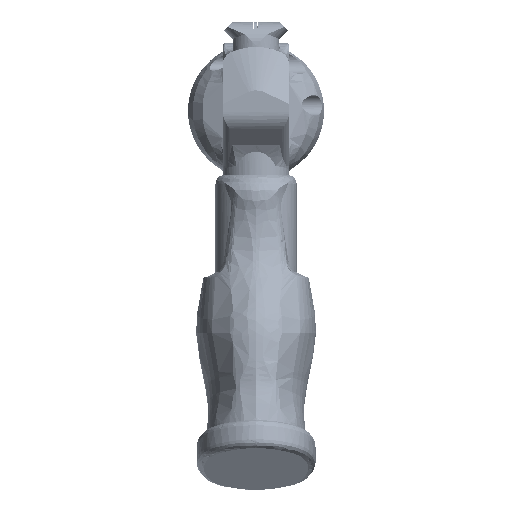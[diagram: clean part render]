
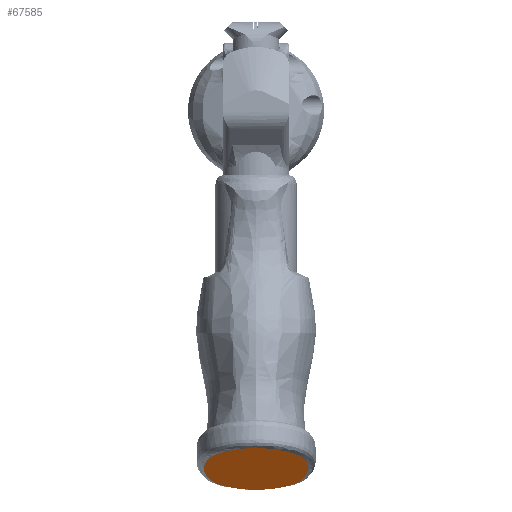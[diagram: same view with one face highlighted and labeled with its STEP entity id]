
A CAD part, left-side view. The second image highlights one B-rep face of the part: STEP entity #67585.
In plain terms, the highlighted planar face has unit normal (-0.259, 0, -0.966).
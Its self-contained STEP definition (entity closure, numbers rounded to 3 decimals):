
#2173=B_SPLINE_CURVE_WITH_KNOTS('',3,(#161349,#161350,#161351,#161352,#161353,
#161354,#161355,#161356,#161357,#161358,#161359,#161360,#161361,#161362,
#161363,#161364,#161365,#161366,#161367,#161368,#161369,#161370,#161371,
#161372,#161373,#161374,#161375,#161376,#161377,#161378,#161379,#161380,
#161381,#161382,#161383,#161384,#161385,#161386,#161387,#161388,#161389,
#161390,#161391),.UNSPECIFIED.,.F.,.F.,(4,2,2,1,1,2,2,2,2,2,1,2,2,2,2,2,
1,2,2,2,1,2,2,4),(0.006,0.019,0.572,
0.597,0.912,1.167,1.831,2.109,
2.578,3.454,3.481,3.884,4.134,
4.709,4.967,5.471,5.557,6.204,
6.731,6.892,6.95,7.028,7.341,
7.351),.UNSPECIFIED.);
#2178=B_SPLINE_CURVE_WITH_KNOTS('',3,(#162170,#162171,#162172,#162173,#162174,
#162175,#162176,#162177,#162178,#162179,#162180,#162181,#162182,#162183,
#162184,#162185,#162186,#162187,#162188,#162189,#162190,#162191,#162192,
#162193,#162194,#162195,#162196,#162197,#162198,#162199,#162200,#162201,
#162202,#162203,#162204,#162205,#162206,#162207,#162208,#162209),
 .UNSPECIFIED.,.F.,.F.,(4,2,2,2,1,2,2,1,2,2,2,1,2,2,2,1,1,2,1,2,2,2,4),
(0.005,0.015,0.356,0.55,
1.005,1.346,1.422,1.811,2.103,
2.274,2.794,3.528,4.506,5.04,
5.1,5.111,5.422,5.851,6.245,
6.541,6.928,7.33,7.342),
 .UNSPECIFIED.);
#7632=PLANE('',#72835);
#10660=FACE_OUTER_BOUND('',#14554,.T.);
#14554=EDGE_LOOP('',(#54560,#54561));
#28957=VERTEX_POINT('',#161347);
#28958=VERTEX_POINT('',#161348);
#38200=EDGE_CURVE('',#28957,#28958,#2173,.T.);
#38205=EDGE_CURVE('',#28958,#28957,#2178,.T.);
#54560=ORIENTED_EDGE('',*,*,#38200,.F.);
#54561=ORIENTED_EDGE('',*,*,#38205,.F.);
#67585=ADVANCED_FACE('',(#10660),#7632,.T.);
#72835=AXIS2_PLACEMENT_3D('',#163135,#83490,#83491);
#83490=DIRECTION('center_axis',(-0.259,0.,
-0.966));
#83491=DIRECTION('ref_axis',(0.,-1.,0.));
#161347=CARTESIAN_POINT('',(32.882,-157.25,88.674));
#161348=CARTESIAN_POINT('',(-20.756,-157.25,103.064));
#161349=CARTESIAN_POINT('Ctrl Pts',(32.882,-157.25,88.674));
#161350=CARTESIAN_POINT('Ctrl Pts',(32.881,-157.207,
88.674));
#161351=CARTESIAN_POINT('Ctrl Pts',(32.879,-157.165,
88.674));
#161352=CARTESIAN_POINT('Ctrl Pts',(32.833,-155.278,88.687));
#161353=CARTESIAN_POINT('Ctrl Pts',(32.449,-153.446,
88.79));
#161354=CARTESIAN_POINT('Ctrl Pts',(31.737,-151.651,
88.981));
#161355=CARTESIAN_POINT('Ctrl Pts',(31.309,-150.596,
89.096));
#161356=CARTESIAN_POINT('Ctrl Pts',(30.365,-148.833,89.349));
#161357=CARTESIAN_POINT('Ctrl Pts',(29.21,-147.352,89.659));
#161358=CARTESIAN_POINT('Ctrl Pts',(27.179,-145.097,
90.204));
#161359=CARTESIAN_POINT('Ctrl Pts',(25.41,-143.763,
90.678));
#161360=CARTESIAN_POINT('Ctrl Pts',(22.707,-142.346,91.403));
#161361=CARTESIAN_POINT('Ctrl Pts',(21.883,-141.976,91.625));
#161362=CARTESIAN_POINT('Ctrl Pts',(19.595,-141.157,
92.238));
#161363=CARTESIAN_POINT('Ctrl Pts',(18.104,-140.785,92.639));
#161364=CARTESIAN_POINT('Ctrl Pts',(13.816,-139.821,
93.789));
#161365=CARTESIAN_POINT('Ctrl Pts',(11.021,-139.412,94.539));
#161366=CARTESIAN_POINT('Ctrl Pts',(8.105,-139.246,
95.321));
#161367=CARTESIAN_POINT('Ctrl Pts',(6.716,-139.171,
95.694));
#161368=CARTESIAN_POINT('Ctrl Pts',(5.323,-139.156,96.068));
#161369=CARTESIAN_POINT('Ctrl Pts',(3.21,-139.215,
96.634));
#161370=CARTESIAN_POINT('Ctrl Pts',(2.405,-139.257,
96.85));
#161371=CARTESIAN_POINT('Ctrl Pts',(-0.254,-139.463,
97.564));
#161372=CARTESIAN_POINT('Ctrl Pts',(-2.091,-139.713,
98.057));
#161373=CARTESIAN_POINT('Ctrl Pts',(-4.746,-140.207,
98.769));
#161374=CARTESIAN_POINT('Ctrl Pts',(-5.561,-140.39,
98.988));
#161375=CARTESIAN_POINT('Ctrl Pts',(-7.944,-141.033,
99.627));
#161376=CARTESIAN_POINT('Ctrl Pts',(-9.486,-141.578,
100.041));
#161377=CARTESIAN_POINT('Ctrl Pts',(-11.184,-142.482,
100.496));
#161378=CARTESIAN_POINT('Ctrl Pts',(-13.267,-143.655,
101.055));
#161379=CARTESIAN_POINT('Ctrl Pts',(-15.122,-145.243,
101.553));
#161380=CARTESIAN_POINT('Ctrl Pts',(-17.614,-148.204,
102.221));
#161381=CARTESIAN_POINT('Ctrl Pts',(-18.556,-149.682,
102.474));
#161382=CARTESIAN_POINT('Ctrl Pts',(-19.536,-151.753,
102.737));
#161383=CARTESIAN_POINT('Ctrl Pts',(-19.748,-152.249,
102.794));
#161384=CARTESIAN_POINT('Ctrl Pts',(-19.999,-152.936,
102.861));
#161385=CARTESIAN_POINT('Ctrl Pts',(-20.144,-153.362,
102.9));
#161386=CARTESIAN_POINT('Ctrl Pts',(-20.271,-153.794,
102.934));
#161387=CARTESIAN_POINT('Ctrl Pts',(-20.592,-155.054,
103.02));
#161388=CARTESIAN_POINT('Ctrl Pts',(-20.733,-156.102,
103.058));
#161389=CARTESIAN_POINT('Ctrl Pts',(-20.755,-157.181,
103.064));
#161390=CARTESIAN_POINT('Ctrl Pts',(-20.755,-157.216,
103.064));
#161391=CARTESIAN_POINT('Ctrl Pts',(-20.756,-157.25,
103.064));
#162170=CARTESIAN_POINT('Ctrl Pts',(-20.756,-157.25,
103.064));
#162171=CARTESIAN_POINT('Ctrl Pts',(-20.755,-157.284,
103.064));
#162172=CARTESIAN_POINT('Ctrl Pts',(-20.755,-157.319,
103.064));
#162173=CARTESIAN_POINT('Ctrl Pts',(-20.731,-158.488,
103.058));
#162174=CARTESIAN_POINT('Ctrl Pts',(-20.566,-159.63,
103.013));
#162175=CARTESIAN_POINT('Ctrl Pts',(-20.09,-161.346,
102.886));
#162176=CARTESIAN_POINT('Ctrl Pts',(-19.87,-161.954,
102.827));
#162177=CARTESIAN_POINT('Ctrl Pts',(-19.017,-163.94,
102.598));
#162178=CARTESIAN_POINT('Ctrl Pts',(-17.697,-166.275,
102.244));
#162179=CARTESIAN_POINT('Ctrl Pts',(-15.982,-168.259,
101.784));
#162180=CARTESIAN_POINT('Ctrl Pts',(-14.995,-169.22,
101.519));
#162181=CARTESIAN_POINT('Ctrl Pts',(-14.812,-169.392,
101.47));
#162182=CARTESIAN_POINT('Ctrl Pts',(-13.674,-170.421,
101.164));
#162183=CARTESIAN_POINT('Ctrl Pts',(-11.848,-171.746,
100.674));
#162184=CARTESIAN_POINT('Ctrl Pts',(-9.863,-172.705,
100.142));
#162185=CARTESIAN_POINT('Ctrl Pts',(-8.467,-173.245,
99.767));
#162186=CARTESIAN_POINT('Ctrl Pts',(-7.946,-173.428,
99.627));
#162187=CARTESIAN_POINT('Ctrl Pts',(-5.808,-174.093,
99.054));
#162188=CARTESIAN_POINT('Ctrl Pts',(-4.141,-174.431,
98.606));
#162189=CARTESIAN_POINT('Ctrl Pts',(-0.107,-175.073,
97.524));
#162190=CARTESIAN_POINT('Ctrl Pts',(5.389,-175.566,
96.05));
#162191=CARTESIAN_POINT('Ctrl Pts',(10.963,-175.11,
94.554));
#162192=CARTESIAN_POINT('Ctrl Pts',(15.784,-174.258,
93.261));
#162193=CARTESIAN_POINT('Ctrl Pts',(17.458,-173.877,
92.812));
#162194=CARTESIAN_POINT('Ctrl Pts',(19.327,-173.376,
92.31));
#162195=CARTESIAN_POINT('Ctrl Pts',(19.515,-173.323,92.26));
#162196=CARTESIAN_POINT('Ctrl Pts',(19.737,-173.257,
92.2));
#162197=CARTESIAN_POINT('Ctrl Pts',(20.746,-172.957,91.93));
#162198=CARTESIAN_POINT('Ctrl Pts',(23.057,-172.074,
91.31));
#162199=CARTESIAN_POINT('Ctrl Pts',(25.138,-170.838,
90.751));
#162200=CARTESIAN_POINT('Ctrl Pts',(27.271,-169.202,
90.179));
#162201=CARTESIAN_POINT('Ctrl Pts',(28.932,-167.617,
89.733));
#162202=CARTESIAN_POINT('Ctrl Pts',(30.246,-165.752,
89.381));
#162203=CARTESIAN_POINT('Ctrl Pts',(31.379,-163.788,
89.077));
#162204=CARTESIAN_POINT('Ctrl Pts',(31.897,-162.583,88.938));
#162205=CARTESIAN_POINT('Ctrl Pts',(32.635,-160.048,
88.74));
#162206=CARTESIAN_POINT('Ctrl Pts',(32.845,-158.717,
88.683));
#162207=CARTESIAN_POINT('Ctrl Pts',(32.879,-157.335,
88.674));
#162208=CARTESIAN_POINT('Ctrl Pts',(32.881,-157.293,
88.674));
#162209=CARTESIAN_POINT('Ctrl Pts',(32.882,-157.25,
88.674));
#163135=CARTESIAN_POINT('Origin',(6.063,-157.388,95.869));
